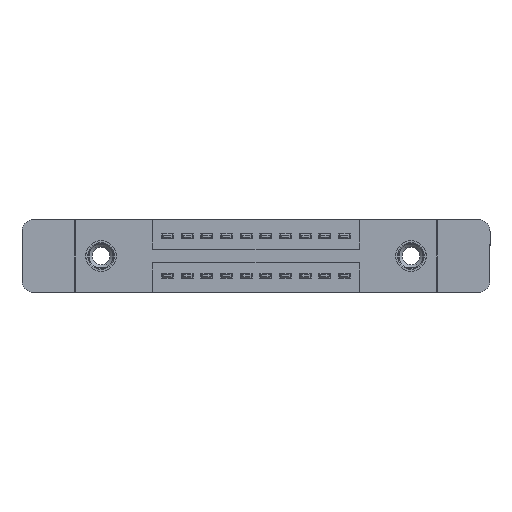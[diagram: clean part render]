
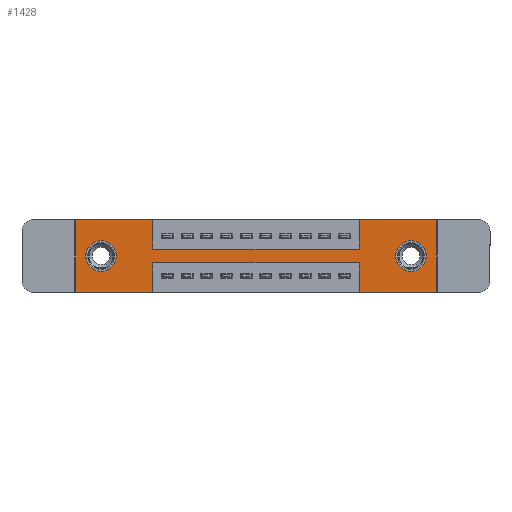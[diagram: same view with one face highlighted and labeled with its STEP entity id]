
A CAD part, front view. The second image highlights one B-rep face of the part: STEP entity #1428.
In plain terms, the highlighted planar face has unit normal (0, -1, 0).
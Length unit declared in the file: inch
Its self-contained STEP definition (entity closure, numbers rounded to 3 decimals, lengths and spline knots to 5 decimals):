
#413 = VERTEX_POINT ( 'NONE', #3661 ) ;
#416 = CIRCLE ( 'NONE', #5257, 0.078 ) ;
#547 = VECTOR ( 'NONE', #8980, 39.37008 ) ;
#709 = CARTESIAN_POINT ( 'NONE',  ( 1.4425, 0., 0. ) ) ;
#789 = ORIENTED_EDGE ( 'NONE', *, *, #16517, .F. ) ;
#1226 = DIRECTION ( 'NONE',  ( 0., 1., 0. ) ) ;
#1261 = EDGE_CURVE ( 'NONE', #16406, #15659, #11221, .T. ) ;
#1277 = AXIS2_PLACEMENT_3D ( 'NONE', #2891, #12237, #4234 ) ;
#1301 = VERTEX_POINT ( 'NONE', #8705 ) ;
#1428 = ADVANCED_FACE ( 'NONE', ( #8679, #5573, #2024 ), #7778, .T. ) ;
#1459 = LINE ( 'NONE', #16220, #11296 ) ;
#1870 = ORIENTED_EDGE ( 'NONE', *, *, #3670, .F. ) ;
#1929 = CIRCLE ( 'NONE', #5855, 0.078 ) ;
#2024 = FACE_OUTER_BOUND ( 'NONE', #15407, .T. ) ;
#2087 = CARTESIAN_POINT ( 'NONE',  ( 1.4425, 0., -0.37 ) ) ;
#2299 = VECTOR ( 'NONE', #6313, 39.37008 ) ;
#2435 = DIRECTION ( 'NONE',  ( -1., 0., 0. ) ) ;
#2617 = EDGE_CURVE ( 'NONE', #15659, #7557, #6136, .T. ) ;
#2891 = CARTESIAN_POINT ( 'NONE',  ( 1.705, 0., -0.185 ) ) ;
#3059 = EDGE_CURVE ( 'NONE', #7557, #9224, #13631, .T. ) ;
#3453 = AXIS2_PLACEMENT_3D ( 'NONE', #9237, #1226, #10598 ) ;
#3571 = VERTEX_POINT ( 'NONE', #5751 ) ;
#3661 = CARTESIAN_POINT ( 'NONE',  ( 1.4425, 0., -0.15 ) ) ;
#3670 = EDGE_CURVE ( 'NONE', #10459, #3571, #5293, .T. ) ;
#3715 = VERTEX_POINT ( 'NONE', #15504 ) ;
#3835 = EDGE_CURVE ( 'NONE', #7086, #13138, #9879, .T. ) ;
#3972 = CARTESIAN_POINT ( 'NONE',  ( 0.13, 0., -0.107 ) ) ;
#4023 = CARTESIAN_POINT ( 'NONE',  ( 1.4425, 0., 0. ) ) ;
#4072 = EDGE_CURVE ( 'NONE', #10200, #10652, #9661, .T. ) ;
#4234 = DIRECTION ( 'NONE',  ( 0., 0., -1. ) ) ;
#4385 = CARTESIAN_POINT ( 'NONE',  ( 0.3925, 0., 0. ) ) ;
#4396 = LINE ( 'NONE', #4833, #10681 ) ;
#4787 = DIRECTION ( 'NONE',  ( -1., 0., 0. ) ) ;
#4833 = CARTESIAN_POINT ( 'NONE',  ( 0.3925, 0., -0.15 ) ) ;
#4882 = VERTEX_POINT ( 'NONE', #16567 ) ;
#4895 = DIRECTION ( 'NONE',  ( 0., 1., 0. ) ) ;
#4960 = ORIENTED_EDGE ( 'NONE', *, *, #9085, .F. ) ;
#5016 = ORIENTED_EDGE ( 'NONE', *, *, #1261, .F. ) ;
#5022 = LINE ( 'NONE', #4023, #15156 ) ;
#5227 = VERTEX_POINT ( 'NONE', #709 ) ;
#5235 = VECTOR ( 'NONE', #2435, 39.37008 ) ;
#5257 = AXIS2_PLACEMENT_3D ( 'NONE', #12877, #4895, #14180 ) ;
#5293 = LINE ( 'NONE', #15166, #11973 ) ;
#5336 = DIRECTION ( 'NONE',  ( 1., 0., 0. ) ) ;
#5429 = LINE ( 'NONE', #15559, #2299 ) ;
#5573 = FACE_BOUND ( 'NONE', #10290, .T. ) ;
#5621 = VECTOR ( 'NONE', #5336, 39.37008 ) ;
#5727 = DIRECTION ( 'NONE',  ( 0., 0., -1. ) ) ;
#5751 = CARTESIAN_POINT ( 'NONE',  ( 1.835, 0., -0.37 ) ) ;
#5855 = AXIS2_PLACEMENT_3D ( 'NONE', #14298, #6329, #15575 ) ;
#5940 = EDGE_CURVE ( 'NONE', #10652, #413, #4396, .T. ) ;
#5950 = EDGE_CURVE ( 'NONE', #13138, #7086, #416, .T. ) ;
#6136 = LINE ( 'NONE', #14078, #16244 ) ;
#6142 = CARTESIAN_POINT ( 'NONE',  ( 0.3925, 0., -0.15 ) ) ;
#6160 = CARTESIAN_POINT ( 'NONE',  ( 0.3925, 0., -0.37 ) ) ;
#6313 = DIRECTION ( 'NONE',  ( -1., 0., 0. ) ) ;
#6329 = DIRECTION ( 'NONE',  ( 0., 1., 0. ) ) ;
#6767 = EDGE_CURVE ( 'NONE', #15766, #10200, #9600, .T. ) ;
#7086 = VERTEX_POINT ( 'NONE', #12901 ) ;
#7380 = DIRECTION ( 'NONE',  ( 0., 0., 1. ) ) ;
#7456 = DIRECTION ( 'NONE',  ( 0., 0., -1. ) ) ;
#7478 = DIRECTION ( 'NONE',  ( 0., -1., 0. ) ) ;
#7482 = CARTESIAN_POINT ( 'NONE',  ( 0., 0., -0.37 ) ) ;
#7557 = VERTEX_POINT ( 'NONE', #15024 ) ;
#7680 = ORIENTED_EDGE ( 'NONE', *, *, #3059, .F. ) ;
#7778 = PLANE ( 'NONE',  #9337 ) ;
#7805 = ORIENTED_EDGE ( 'NONE', *, *, #12705, .T. ) ;
#7972 = EDGE_LOOP ( 'NONE', ( #7805, #12885 ) ) ;
#8342 = DIRECTION ( 'NONE',  ( 1., 0., 0. ) ) ;
#8679 = FACE_BOUND ( 'NONE', #7972, .T. ) ;
#8705 = CARTESIAN_POINT ( 'NONE',  ( 0., 0., -0.37 ) ) ;
#8858 = ORIENTED_EDGE ( 'NONE', *, *, #5940, .F. ) ;
#8980 = DIRECTION ( 'NONE',  ( 0., 0., 1. ) ) ;
#9085 = EDGE_CURVE ( 'NONE', #1301, #15766, #17076, .T. ) ;
#9184 = LINE ( 'NONE', #13031, #5235 ) ;
#9224 = VERTEX_POINT ( 'NONE', #15695 ) ;
#9237 = CARTESIAN_POINT ( 'NONE',  ( 0.13, 0., -0.185 ) ) ;
#9337 = AXIS2_PLACEMENT_3D ( 'NONE', #7482, #7478, #7456 ) ;
#9475 = CARTESIAN_POINT ( 'NONE',  ( 1.4425, 0., -0.22 ) ) ;
#9600 = LINE ( 'NONE', #10654, #5621 ) ;
#9661 = LINE ( 'NONE', #4385, #15797 ) ;
#9717 = ORIENTED_EDGE ( 'NONE', *, *, #6767, .F. ) ;
#9844 = CARTESIAN_POINT ( 'NONE',  ( 1.835, 0., 0. ) ) ;
#9879 = CIRCLE ( 'NONE', #3453, 0.078 ) ;
#9985 = ORIENTED_EDGE ( 'NONE', *, *, #5950, .T. ) ;
#10014 = DIRECTION ( 'NONE',  ( 0., 0., -1. ) ) ;
#10061 = CARTESIAN_POINT ( 'NONE',  ( 1.4425, 0., -0.37 ) ) ;
#10200 = VERTEX_POINT ( 'NONE', #16168 ) ;
#10290 = EDGE_LOOP ( 'NONE', ( #9985, #15700 ) ) ;
#10459 = VERTEX_POINT ( 'NONE', #9844 ) ;
#10598 = DIRECTION ( 'NONE',  ( 0., 0., 1. ) ) ;
#10652 = VERTEX_POINT ( 'NONE', #6142 ) ;
#10654 = CARTESIAN_POINT ( 'NONE',  ( 0., 0., 0. ) ) ;
#10681 = VECTOR ( 'NONE', #11494, 39.37008 ) ;
#10967 = ORIENTED_EDGE ( 'NONE', *, *, #4072, .F. ) ;
#11221 = LINE ( 'NONE', #10061, #547 ) ;
#11296 = VECTOR ( 'NONE', #8342, 39.37008 ) ;
#11494 = DIRECTION ( 'NONE',  ( 1., 0., 0. ) ) ;
#11787 = EDGE_CURVE ( 'NONE', #4882, #3715, #1929, .T. ) ;
#11964 = DIRECTION ( 'NONE',  ( 0., 0., 1. ) ) ;
#11973 = VECTOR ( 'NONE', #10014, 39.37008 ) ;
#12237 = DIRECTION ( 'NONE',  ( 0., 1., 0. ) ) ;
#12591 = ORIENTED_EDGE ( 'NONE', *, *, #12800, .F. ) ;
#12705 = EDGE_CURVE ( 'NONE', #3715, #4882, #15967, .T. ) ;
#12800 = EDGE_CURVE ( 'NONE', #5227, #10459, #1459, .T. ) ;
#12877 = CARTESIAN_POINT ( 'NONE',  ( 0.13, 0., -0.185 ) ) ;
#12885 = ORIENTED_EDGE ( 'NONE', *, *, #11787, .T. ) ;
#12901 = CARTESIAN_POINT ( 'NONE',  ( 0.13, 0., -0.263 ) ) ;
#13031 = CARTESIAN_POINT ( 'NONE',  ( 0., 0., -0.37 ) ) ;
#13138 = VERTEX_POINT ( 'NONE', #3972 ) ;
#13631 = LINE ( 'NONE', #6160, #17023 ) ;
#13674 = VECTOR ( 'NONE', #7380, 39.37008 ) ;
#13705 = EDGE_CURVE ( 'NONE', #3571, #16406, #9184, .T. ) ;
#13740 = CARTESIAN_POINT ( 'NONE',  ( 0., 0., 0. ) ) ;
#14078 = CARTESIAN_POINT ( 'NONE',  ( 0.3925, 0., -0.22 ) ) ;
#14180 = DIRECTION ( 'NONE',  ( 0., 0., 1. ) ) ;
#14218 = ORIENTED_EDGE ( 'NONE', *, *, #16096, .F. ) ;
#14298 = CARTESIAN_POINT ( 'NONE',  ( 1.705, 0., -0.185 ) ) ;
#15024 = CARTESIAN_POINT ( 'NONE',  ( 0.3925, 0., -0.22 ) ) ;
#15156 = VECTOR ( 'NONE', #11964, 39.37008 ) ;
#15166 = CARTESIAN_POINT ( 'NONE',  ( 1.835, 0., 0. ) ) ;
#15407 = EDGE_LOOP ( 'NONE', ( #7680, #16582, #5016, #16750, #1870, #12591, #14218, #8858, #10967, #9717, #4960, #789 ) ) ;
#15504 = CARTESIAN_POINT ( 'NONE',  ( 1.705, 0., -0.107 ) ) ;
#15559 = CARTESIAN_POINT ( 'NONE',  ( 0., 0., -0.37 ) ) ;
#15575 = DIRECTION ( 'NONE',  ( 0., 0., -1. ) ) ;
#15659 = VERTEX_POINT ( 'NONE', #9475 ) ;
#15695 = CARTESIAN_POINT ( 'NONE',  ( 0.3925, 0., -0.37 ) ) ;
#15700 = ORIENTED_EDGE ( 'NONE', *, *, #3835, .T. ) ;
#15766 = VERTEX_POINT ( 'NONE', #13740 ) ;
#15797 = VECTOR ( 'NONE', #5727, 39.37008 ) ;
#15967 = CIRCLE ( 'NONE', #1277, 0.078 ) ;
#16096 = EDGE_CURVE ( 'NONE', #413, #5227, #5022, .T. ) ;
#16168 = CARTESIAN_POINT ( 'NONE',  ( 0.3925, 0., 0. ) ) ;
#16220 = CARTESIAN_POINT ( 'NONE',  ( 0., 0., 0. ) ) ;
#16244 = VECTOR ( 'NONE', #4787, 39.37008 ) ;
#16406 = VERTEX_POINT ( 'NONE', #2087 ) ;
#16517 = EDGE_CURVE ( 'NONE', #9224, #1301, #5429, .T. ) ;
#16567 = CARTESIAN_POINT ( 'NONE',  ( 1.705, 0., -0.263 ) ) ;
#16582 = ORIENTED_EDGE ( 'NONE', *, *, #2617, .F. ) ;
#16583 = CARTESIAN_POINT ( 'NONE',  ( 0., 0., 0. ) ) ;
#16684 = DIRECTION ( 'NONE',  ( 0., 0., -1. ) ) ;
#16750 = ORIENTED_EDGE ( 'NONE', *, *, #13705, .F. ) ;
#17023 = VECTOR ( 'NONE', #16684, 39.37008 ) ;
#17076 = LINE ( 'NONE', #16583, #13674 ) ;
